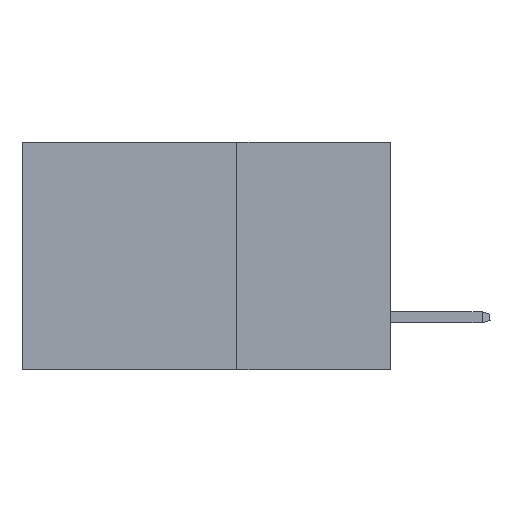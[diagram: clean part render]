
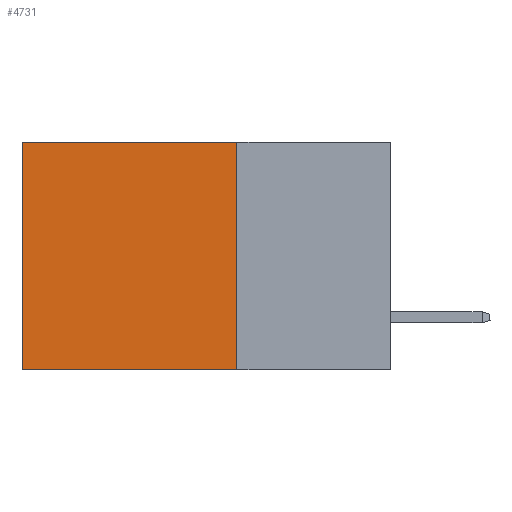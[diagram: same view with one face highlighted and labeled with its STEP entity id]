
A CAD part, left-side view. The second image highlights one B-rep face of the part: STEP entity #4731.
In plain terms, the highlighted planar face has unit normal (-1, 0, 0).
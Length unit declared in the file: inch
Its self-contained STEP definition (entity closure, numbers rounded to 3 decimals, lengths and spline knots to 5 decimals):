
#69 = ORIENTED_EDGE ( 'NONE', *, *, #6167, .T. ) ;
#2051 = VECTOR ( 'NONE', #19827, 39.37008 ) ;
#2164 = ORIENTED_EDGE ( 'NONE', *, *, #5925, .F. ) ;
#2565 = DIRECTION ( 'NONE',  ( 0., 0., -1. ) ) ;
#2752 = CARTESIAN_POINT ( 'NONE',  ( 0.2875, 0.25, 0. ) ) ;
#3302 = CARTESIAN_POINT ( 'NONE',  ( 0.2875, 0.25, -0.37 ) ) ;
#3377 = DIRECTION ( 'NONE',  ( 0., 1., 0. ) ) ;
#3420 = VECTOR ( 'NONE', #8733, 39.37008 ) ;
#4731 = ADVANCED_FACE ( 'NONE', ( #10396 ), #7227, .F. ) ;
#4806 = VERTEX_POINT ( 'NONE', #17328 ) ;
#5876 = LINE ( 'NONE', #19031, #7337 ) ;
#5925 = EDGE_CURVE ( 'NONE', #17570, #8622, #5876, .T. ) ;
#6063 = AXIS2_PLACEMENT_3D ( 'NONE', #2752, #10423, #2565 ) ;
#6167 = EDGE_CURVE ( 'NONE', #17570, #10197, #6339, .T. ) ;
#6339 = LINE ( 'NONE', #11999, #3420 ) ;
#7227 = PLANE ( 'NONE',  #6063 ) ;
#7337 = VECTOR ( 'NONE', #10871, 39.37008 ) ;
#8307 = CARTESIAN_POINT ( 'NONE',  ( 0.2875, 0.6, 0. ) ) ;
#8622 = VERTEX_POINT ( 'NONE', #14552 ) ;
#8733 = DIRECTION ( 'NONE',  ( 0., 1., 0. ) ) ;
#10197 = VERTEX_POINT ( 'NONE', #15925 ) ;
#10396 = FACE_OUTER_BOUND ( 'NONE', #15937, .T. ) ;
#10423 = DIRECTION ( 'NONE',  ( 1., 0., 0. ) ) ;
#10871 = DIRECTION ( 'NONE',  ( 0., 0., -1. ) ) ;
#11782 = CARTESIAN_POINT ( 'NONE',  ( 0.2875, 0.25, 0. ) ) ;
#11838 = ORIENTED_EDGE ( 'NONE', *, *, #15885, .T. ) ;
#11999 = CARTESIAN_POINT ( 'NONE',  ( 0.2875, 0.25, 0. ) ) ;
#12061 = LINE ( 'NONE', #3302, #16798 ) ;
#13870 = ORIENTED_EDGE ( 'NONE', *, *, #19624, .F. ) ;
#14552 = CARTESIAN_POINT ( 'NONE',  ( 0.2875, 0.25, -0.37 ) ) ;
#15885 = EDGE_CURVE ( 'NONE', #10197, #4806, #18181, .T. ) ;
#15925 = CARTESIAN_POINT ( 'NONE',  ( 0.2875, 0.6, 0. ) ) ;
#15937 = EDGE_LOOP ( 'NONE', ( #11838, #13870, #2164, #69 ) ) ;
#16798 = VECTOR ( 'NONE', #3377, 39.37008 ) ;
#17328 = CARTESIAN_POINT ( 'NONE',  ( 0.2875, 0.6, -0.37 ) ) ;
#17570 = VERTEX_POINT ( 'NONE', #11782 ) ;
#18181 = LINE ( 'NONE', #8307, #2051 ) ;
#19031 = CARTESIAN_POINT ( 'NONE',  ( 0.2875, 0.25, 0. ) ) ;
#19624 = EDGE_CURVE ( 'NONE', #8622, #4806, #12061, .T. ) ;
#19827 = DIRECTION ( 'NONE',  ( 0., 0., -1. ) ) ;
